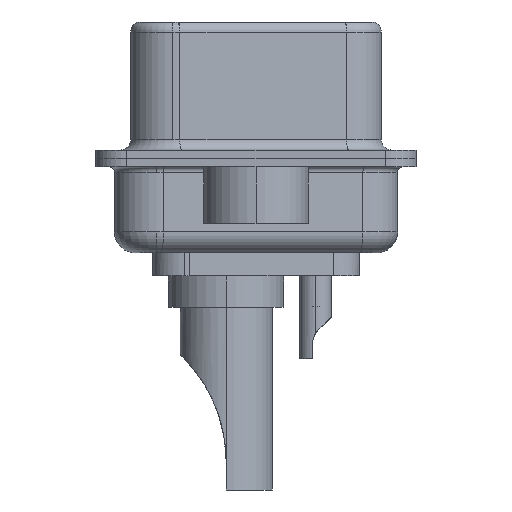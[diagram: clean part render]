
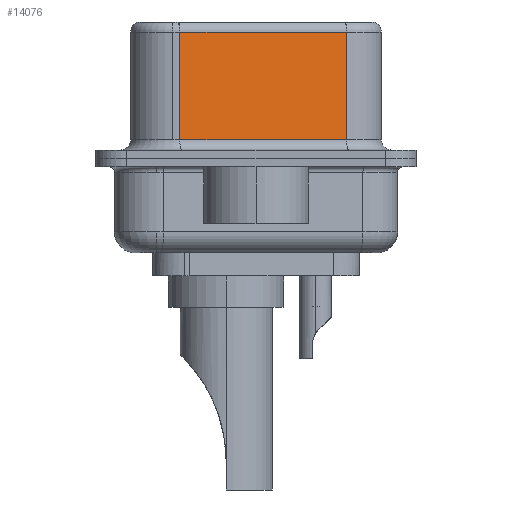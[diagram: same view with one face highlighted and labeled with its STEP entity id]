
A CAD part, left-side view. The second image highlights one B-rep face of the part: STEP entity #14076.
In plain terms, the highlighted planar face has unit normal (-0.985, -0.174, 0).
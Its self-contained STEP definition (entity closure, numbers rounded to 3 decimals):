
#2 = EDGE_LOOP ( 'NONE', ( #1576, #18945, #2367, #15547 ) ) ;
#52 = VERTEX_POINT ( 'NONE', #1747 ) ;
#975 = DIRECTION ( 'NONE',  ( 0.985, 0.174, 0. ) ) ;
#1576 = ORIENTED_EDGE ( 'NONE', *, *, #4673, .F. ) ;
#1747 = CARTESIAN_POINT ( 'NONE',  ( 5.132, -4.322, 6.02 ) ) ;
#1846 = CARTESIAN_POINT ( 'NONE',  ( 3.73, 3.628, 6.02 ) ) ;
#1866 = CARTESIAN_POINT ( 'NONE',  ( 5.132, -4.322, 0.9 ) ) ;
#2283 = CARTESIAN_POINT ( 'NONE',  ( 5.132, -4.322, 0.9 ) ) ;
#2367 = ORIENTED_EDGE ( 'NONE', *, *, #14221, .T. ) ;
#2430 = VERTEX_POINT ( 'NONE', #1846 ) ;
#3955 = VECTOR ( 'NONE', #8022, 1000. ) ;
#4140 = EDGE_CURVE ( 'NONE', #17430, #10409, #13980, .T. ) ;
#4517 = LINE ( 'NONE', #7637, #8401 ) ;
#4673 = EDGE_CURVE ( 'NONE', #52, #10409, #9546, .T. ) ;
#7637 = CARTESIAN_POINT ( 'NONE',  ( 5.132, -4.322, 6.02 ) ) ;
#8022 = DIRECTION ( 'NONE',  ( 0., 0., -1. ) ) ;
#8401 = VECTOR ( 'NONE', #17584, 1000. ) ;
#9060 = VECTOR ( 'NONE', #17234, 1000. ) ;
#9546 = LINE ( 'NONE', #17965, #13960 ) ;
#10409 = VERTEX_POINT ( 'NONE', #1866 ) ;
#10914 = PLANE ( 'NONE',  #13598 ) ;
#11077 = EDGE_CURVE ( 'NONE', #52, #2430, #4517, .T. ) ;
#11673 = CARTESIAN_POINT ( 'NONE',  ( 3.73, 3.628, 0.9 ) ) ;
#12590 = DIRECTION ( 'NONE',  ( -0.174, 0.985, 0. ) ) ;
#13598 = AXIS2_PLACEMENT_3D ( 'NONE', #15787, #975, #12590 ) ;
#13960 = VECTOR ( 'NONE', #19633, 1000. ) ;
#13980 = LINE ( 'NONE', #2283, #9060 ) ;
#14076 = ADVANCED_FACE ( 'NONE', ( #19754 ), #10914, .F. ) ;
#14221 = EDGE_CURVE ( 'NONE', #2430, #17430, #16643, .T. ) ;
#15547 = ORIENTED_EDGE ( 'NONE', *, *, #4140, .T. ) ;
#15787 = CARTESIAN_POINT ( 'NONE',  ( 5.132, -4.322, 6.52 ) ) ;
#16643 = LINE ( 'NONE', #17944, #3955 ) ;
#17234 = DIRECTION ( 'NONE',  ( 0.174, -0.985, 0. ) ) ;
#17430 = VERTEX_POINT ( 'NONE', #11673 ) ;
#17584 = DIRECTION ( 'NONE',  ( -0.174, 0.985, 0. ) ) ;
#17944 = CARTESIAN_POINT ( 'NONE',  ( 3.73, 3.628, 6.52 ) ) ;
#17965 = CARTESIAN_POINT ( 'NONE',  ( 5.132, -4.322, 6.52 ) ) ;
#18945 = ORIENTED_EDGE ( 'NONE', *, *, #11077, .T. ) ;
#19633 = DIRECTION ( 'NONE',  ( 0., 0., -1. ) ) ;
#19754 = FACE_OUTER_BOUND ( 'NONE', #2, .T. ) ;
